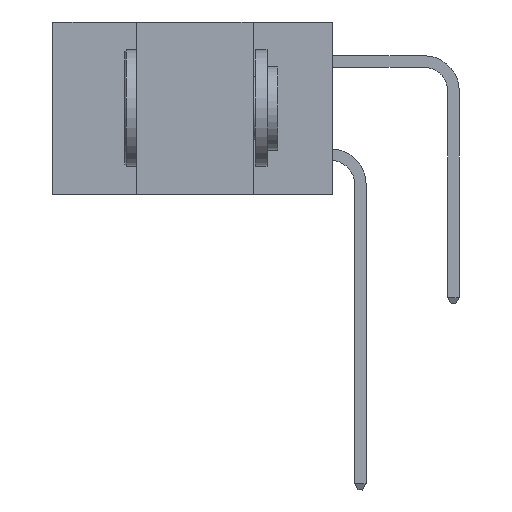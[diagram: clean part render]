
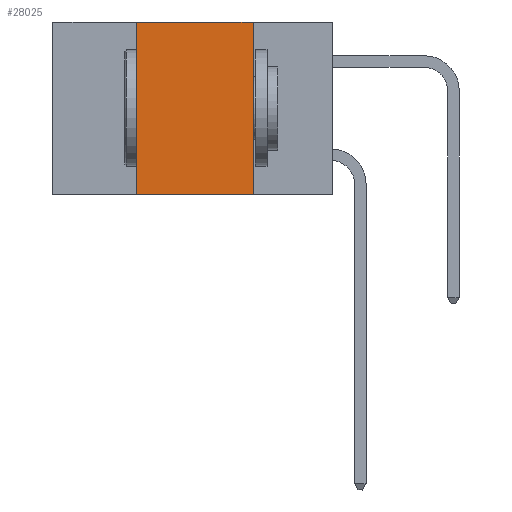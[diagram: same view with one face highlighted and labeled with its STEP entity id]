
A CAD part, left-side view. The second image highlights one B-rep face of the part: STEP entity #28025.
In plain terms, the highlighted planar face has unit normal (-1, 0, 0).
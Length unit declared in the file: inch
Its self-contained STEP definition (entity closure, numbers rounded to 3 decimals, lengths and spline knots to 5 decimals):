
#1290 = ORIENTED_EDGE ( 'NONE', *, *, #6004, .F. ) ;
#1313 = DIRECTION ( 'NONE',  ( 1., 0., 0. ) ) ;
#1803 = AXIS2_PLACEMENT_3D ( 'NONE', #11834, #1313, #19576 ) ;
#2030 = CARTESIAN_POINT ( 'NONE',  ( 0., 0.17, 0. ) ) ;
#3866 = PLANE ( 'NONE',  #1803 ) ;
#4717 = DIRECTION ( 'NONE',  ( 0., 0., -1. ) ) ;
#6004 = EDGE_CURVE ( 'NONE', #15286, #7344, #19148, .T. ) ;
#7264 = DIRECTION ( 'NONE',  ( 0., -1., 0. ) ) ;
#7344 = VERTEX_POINT ( 'NONE', #20991 ) ;
#8366 = CARTESIAN_POINT ( 'NONE',  ( 0., 0.6, -0.37 ) ) ;
#9583 = CARTESIAN_POINT ( 'NONE',  ( 0., 0.42, 0. ) ) ;
#9805 = LINE ( 'NONE', #8366, #15076 ) ;
#11359 = DIRECTION ( 'NONE',  ( 0., 0., 1. ) ) ;
#11834 = CARTESIAN_POINT ( 'NONE',  ( 0., 0.6, 0. ) ) ;
#12215 = LINE ( 'NONE', #2030, #24947 ) ;
#12409 = EDGE_CURVE ( 'NONE', #7344, #31922, #33084, .T. ) ;
#14993 = CARTESIAN_POINT ( 'NONE',  ( 0., 0.6, 0. ) ) ;
#15076 = VECTOR ( 'NONE', #23701, 39.37008 ) ;
#15273 = ORIENTED_EDGE ( 'NONE', *, *, #26598, .T. ) ;
#15286 = VERTEX_POINT ( 'NONE', #23197 ) ;
#16197 = CARTESIAN_POINT ( 'NONE',  ( 0., 0.17, -0.37 ) ) ;
#18464 = ORIENTED_EDGE ( 'NONE', *, *, #25590, .F. ) ;
#19148 = LINE ( 'NONE', #9583, #32455 ) ;
#19576 = DIRECTION ( 'NONE',  ( 0., 0., -1. ) ) ;
#20991 = CARTESIAN_POINT ( 'NONE',  ( 0., 0.42, 0. ) ) ;
#21246 = VERTEX_POINT ( 'NONE', #16197 ) ;
#23197 = CARTESIAN_POINT ( 'NONE',  ( 0., 0.42, -0.37 ) ) ;
#23701 = DIRECTION ( 'NONE',  ( 0., -1., 0. ) ) ;
#24947 = VECTOR ( 'NONE', #4717, 39.37008 ) ;
#25240 = FACE_OUTER_BOUND ( 'NONE', #30487, .T. ) ;
#25590 = EDGE_CURVE ( 'NONE', #31922, #21246, #12215, .T. ) ;
#26598 = EDGE_CURVE ( 'NONE', #15286, #21246, #9805, .T. ) ;
#28025 = ADVANCED_FACE ( 'NONE', ( #25240 ), #3866, .F. ) ;
#30487 = EDGE_LOOP ( 'NONE', ( #18464, #30649, #1290, #15273 ) ) ;
#30649 = ORIENTED_EDGE ( 'NONE', *, *, #12409, .F. ) ;
#31556 = VECTOR ( 'NONE', #7264, 39.37008 ) ;
#31922 = VERTEX_POINT ( 'NONE', #32671 ) ;
#32455 = VECTOR ( 'NONE', #11359, 39.37008 ) ;
#32671 = CARTESIAN_POINT ( 'NONE',  ( 0., 0.17, 0. ) ) ;
#33084 = LINE ( 'NONE', #14993, #31556 ) ;
